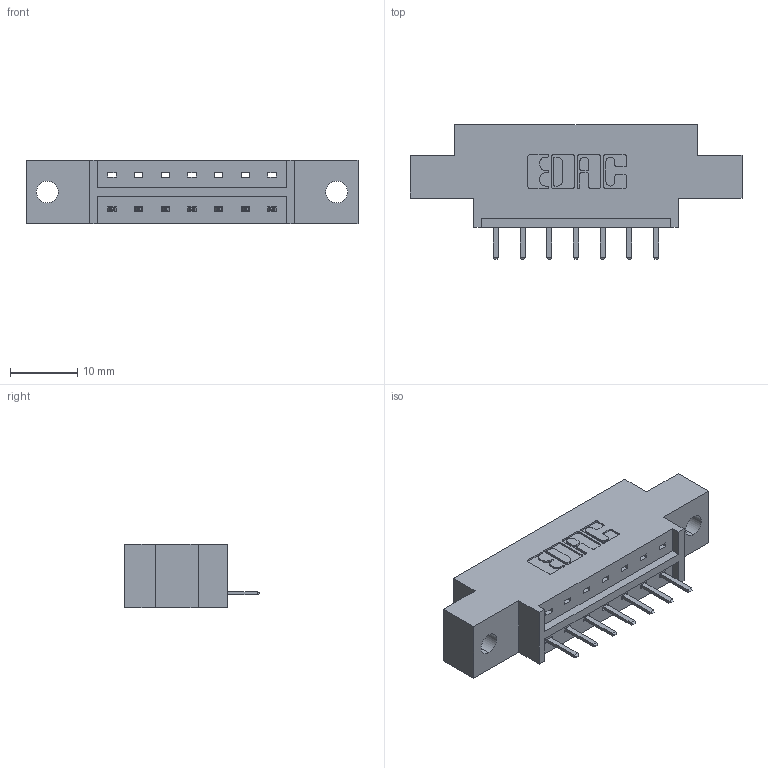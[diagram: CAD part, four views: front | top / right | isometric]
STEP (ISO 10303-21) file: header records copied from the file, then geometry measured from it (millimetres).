
FILE_DESCRIPTION (( 'STEP AP203' ), '1' );
FILE_NAME ('333-007-520-602.STEP', '2018-07-31T21:31:29', ( '' ), ( '' ), 'SwSTEP 2.0', 'SolidWorks 2016', '' );
FILE_SCHEMA (( 'CONFIG_CONTROL_DESIGN' ));
Length unit declared in the file: inch
Products named in the file (3): 333 Part_Offset - .128 Dia; 333-007-520-602; 345-292-001_345-293-120
Assembly tree (8 placements, depth 2):
  333-007-520-602
    333 Part_Offset - .128 Dia
    345-292-001_345-293-120  x7
Bounding box: 49.28 x 20.02 x 9.4 mm (x, y, z)
Volume: 4372.9 mm3; surface area: 4357.4 mm2
Topology: 8 solids, 8 shells, 552 faces, 1611 edges, 1054 vertices
Faces by surface type: plane 382, cylinder 170
Entity records: 9055 total; most frequent: CARTESIAN_POINT 1587, ORIENTED_EDGE 1518, DIRECTION 1397, EDGE_CURVE 759, VECTOR 627, LINE 627, VERTEX_POINT 502, AXIS2_PLACEMENT_3D 385
